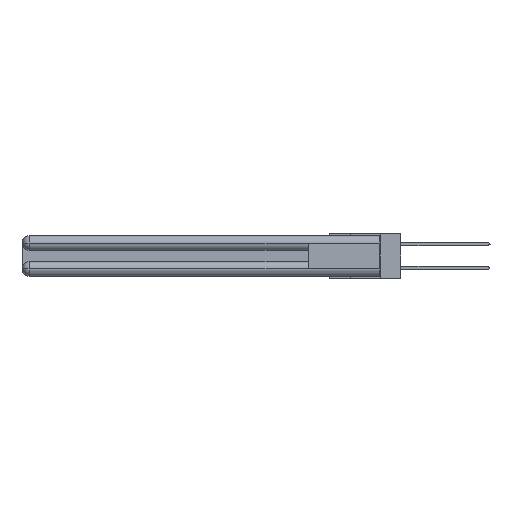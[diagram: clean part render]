
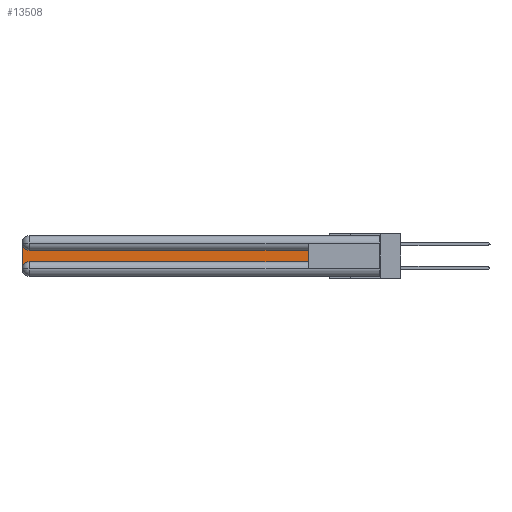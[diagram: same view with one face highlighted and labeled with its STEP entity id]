
A CAD part, left-side view. The second image highlights one B-rep face of the part: STEP entity #13508.
In plain terms, the highlighted planar face has unit normal (-1, 0, 0).
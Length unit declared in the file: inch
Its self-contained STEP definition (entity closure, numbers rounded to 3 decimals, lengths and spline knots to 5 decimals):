
#110 = VERTEX_POINT ( 'NONE', #8128 ) ;
#514 = VERTEX_POINT ( 'NONE', #12611 ) ;
#606 = DIRECTION ( 'NONE',  ( 0., 0., 1. ) ) ;
#751 = VERTEX_POINT ( 'NONE', #26693 ) ;
#1128 = DIRECTION ( 'NONE',  ( 0., 0., -1. ) ) ;
#1283 = AXIS2_PLACEMENT_3D ( 'NONE', #4341, #28857, #9485 ) ;
#3987 = ORIENTED_EDGE ( 'NONE', *, *, #6920, .T. ) ;
#4341 = CARTESIAN_POINT ( 'NONE',  ( 0.075, 3., -0.1225 ) ) ;
#4881 = DIRECTION ( 'NONE',  ( 0., -1., 0. ) ) ;
#5760 = VECTOR ( 'NONE', #21149, 39.37008 ) ;
#6477 = CARTESIAN_POINT ( 'NONE',  ( 0.075, 0.6, -0.1225 ) ) ;
#6825 = CARTESIAN_POINT ( 'NONE',  ( 0.075, 2.94, -0.0625 ) ) ;
#6920 = EDGE_CURVE ( 'NONE', #30068, #514, #23014, .T. ) ;
#7143 = DIRECTION ( 'NONE',  ( 0., 0., -1. ) ) ;
#7488 = ORIENTED_EDGE ( 'NONE', *, *, #10121, .T. ) ;
#8128 = CARTESIAN_POINT ( 'NONE',  ( 0.075, 0.6, -0.2175 ) ) ;
#9261 = ORIENTED_EDGE ( 'NONE', *, *, #11365, .T. ) ;
#9485 = DIRECTION ( 'NONE',  ( 0., 0., -1. ) ) ;
#9504 = DIRECTION ( 'NONE',  ( 1., 0., 0. ) ) ;
#9632 = LINE ( 'NONE', #15333, #10412 ) ;
#10121 = EDGE_CURVE ( 'NONE', #514, #17484, #26679, .T. ) ;
#10412 = VECTOR ( 'NONE', #606, 39.37008 ) ;
#11365 = EDGE_CURVE ( 'NONE', #17484, #17186, #20808, .T. ) ;
#11717 = PLANE ( 'NONE',  #1283 ) ;
#12570 = DIRECTION ( 'NONE',  ( 0., 0., -1. ) ) ;
#12611 = CARTESIAN_POINT ( 'NONE',  ( 0.075, 2.94, -0.1225 ) ) ;
#13334 = CARTESIAN_POINT ( 'NONE',  ( 0.075, 3., -0.2775 ) ) ;
#13508 = ADVANCED_FACE ( 'NONE', ( #31103 ), #11717, .F. ) ;
#13592 = CARTESIAN_POINT ( 'NONE',  ( 0.075, 2.94, -0.2775 ) ) ;
#15333 = CARTESIAN_POINT ( 'NONE',  ( 0.075, 0.6, -0.2175 ) ) ;
#16015 = ORIENTED_EDGE ( 'NONE', *, *, #17014, .T. ) ;
#17014 = EDGE_CURVE ( 'NONE', #751, #110, #30539, .T. ) ;
#17186 = VERTEX_POINT ( 'NONE', #13334 ) ;
#17484 = VERTEX_POINT ( 'NONE', #19491 ) ;
#19491 = CARTESIAN_POINT ( 'NONE',  ( 0.075, 3., -0.0625 ) ) ;
#20808 = LINE ( 'NONE', #22341, #31628 ) ;
#21149 = DIRECTION ( 'NONE',  ( 0., 1., 0. ) ) ;
#21507 = EDGE_CURVE ( 'NONE', #17186, #751, #25836, .T. ) ;
#22334 = EDGE_LOOP ( 'NONE', ( #3987, #7488, #9261, #24308, #16015, #24639 ) ) ;
#22341 = CARTESIAN_POINT ( 'NONE',  ( 0.075, 3., -0.2175 ) ) ;
#23014 = LINE ( 'NONE', #6477, #5760 ) ;
#23053 = DIRECTION ( 'NONE',  ( 1., 0., 0. ) ) ;
#24308 = ORIENTED_EDGE ( 'NONE', *, *, #21507, .T. ) ;
#24639 = ORIENTED_EDGE ( 'NONE', *, *, #30691, .T. ) ;
#24732 = CARTESIAN_POINT ( 'NONE',  ( 0.075, 0.6, -0.2175 ) ) ;
#25836 = CIRCLE ( 'NONE', #26520, 0.06 ) ;
#26520 = AXIS2_PLACEMENT_3D ( 'NONE', #13592, #23053, #1128 ) ;
#26679 = CIRCLE ( 'NONE', #31293, 0.06 ) ;
#26693 = CARTESIAN_POINT ( 'NONE',  ( 0.075, 2.94, -0.2175 ) ) ;
#28677 = CARTESIAN_POINT ( 'NONE',  ( 0.075, 0.6, -0.1225 ) ) ;
#28857 = DIRECTION ( 'NONE',  ( 1., 0., 0. ) ) ;
#30068 = VERTEX_POINT ( 'NONE', #28677 ) ;
#30539 = LINE ( 'NONE', #24732, #31667 ) ;
#30691 = EDGE_CURVE ( 'NONE', #110, #30068, #9632, .T. ) ;
#31103 = FACE_OUTER_BOUND ( 'NONE', #22334, .T. ) ;
#31293 = AXIS2_PLACEMENT_3D ( 'NONE', #6825, #9504, #7143 ) ;
#31628 = VECTOR ( 'NONE', #12570, 39.37008 ) ;
#31667 = VECTOR ( 'NONE', #4881, 39.37008 ) ;
